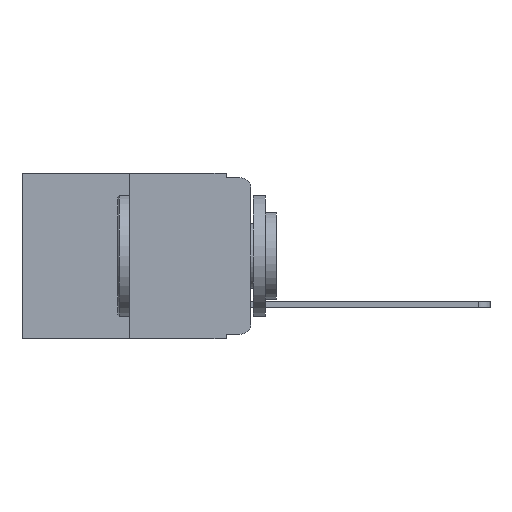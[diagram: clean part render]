
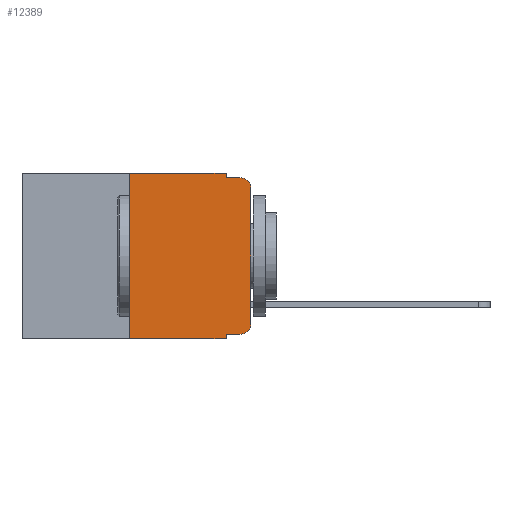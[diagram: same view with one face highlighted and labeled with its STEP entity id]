
A CAD part, left-side view. The second image highlights one B-rep face of the part: STEP entity #12389.
In plain terms, the highlighted planar face has unit normal (-1, 0, 0).
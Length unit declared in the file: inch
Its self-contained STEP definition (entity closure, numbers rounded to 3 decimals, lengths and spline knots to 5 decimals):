
#187 = ORIENTED_EDGE ( 'NONE', *, *, #15981, .F. ) ;
#561 = VECTOR ( 'NONE', #2764, 39.37008 ) ;
#1477 = DIRECTION ( 'NONE',  ( 0., 0., -1. ) ) ;
#1606 = ORIENTED_EDGE ( 'NONE', *, *, #15939, .F. ) ;
#1627 = LINE ( 'NONE', #7523, #6175 ) ;
#1663 = EDGE_CURVE ( 'NONE', #6163, #7898, #3650, .T. ) ;
#1715 = CARTESIAN_POINT ( 'NONE',  ( 0., 0.051, -0.01 ) ) ;
#2299 = CARTESIAN_POINT ( 'NONE',  ( 0., 0.051, -0.343 ) ) ;
#2764 = DIRECTION ( 'NONE',  ( 0., 0., -1. ) ) ;
#3650 = LINE ( 'NONE', #5828, #14278 ) ;
#4396 = ORIENTED_EDGE ( 'NONE', *, *, #6915, .F. ) ;
#5014 = VECTOR ( 'NONE', #7678, 39.37008 ) ;
#5183 = CARTESIAN_POINT ( 'NONE',  ( 0., 0., -0.313 ) ) ;
#5252 = EDGE_CURVE ( 'NONE', #21547, #19564, #20671, .T. ) ;
#5579 = ORIENTED_EDGE ( 'NONE', *, *, #14327, .T. ) ;
#5751 = DIRECTION ( 'NONE',  ( 0., -1., 0. ) ) ;
#5796 = CARTESIAN_POINT ( 'NONE',  ( 0., 0.25, 0. ) ) ;
#5828 = CARTESIAN_POINT ( 'NONE',  ( 0., 0.473, 0. ) ) ;
#5859 = LINE ( 'NONE', #10285, #561 ) ;
#5988 = LINE ( 'NONE', #23269, #15465 ) ;
#6163 = VERTEX_POINT ( 'NONE', #21907 ) ;
#6175 = VECTOR ( 'NONE', #9389, 39.37008 ) ;
#6274 = DIRECTION ( 'NONE',  ( 0., -1., 0. ) ) ;
#6359 = CARTESIAN_POINT ( 'NONE',  ( 0., 0., 0. ) ) ;
#6886 = CARTESIAN_POINT ( 'NONE',  ( 0., 0.051, -0.333 ) ) ;
#6915 = EDGE_CURVE ( 'NONE', #8893, #14971, #8928, .T. ) ;
#7220 = CARTESIAN_POINT ( 'NONE',  ( 0., 0.473, 0. ) ) ;
#7337 = CARTESIAN_POINT ( 'NONE',  ( 0., 0.25, -0.343 ) ) ;
#7523 = CARTESIAN_POINT ( 'NONE',  ( 0., 0.051, 0. ) ) ;
#7678 = DIRECTION ( 'NONE',  ( 0., 0., 1. ) ) ;
#7898 = VERTEX_POINT ( 'NONE', #15655 ) ;
#7917 = LINE ( 'NONE', #14983, #12435 ) ;
#8893 = VERTEX_POINT ( 'NONE', #1715 ) ;
#8928 = LINE ( 'NONE', #17516, #18314 ) ;
#9149 = DIRECTION ( 'NONE',  ( -1., 0., 0. ) ) ;
#9245 = DIRECTION ( 'NONE',  ( -1., 0., 0. ) ) ;
#9276 = VERTEX_POINT ( 'NONE', #18692 ) ;
#9389 = DIRECTION ( 'NONE',  ( 0., 0., -1. ) ) ;
#10231 = DIRECTION ( 'NONE',  ( 0., 0., 1. ) ) ;
#10285 = CARTESIAN_POINT ( 'NONE',  ( 0., 0.051, 0. ) ) ;
#10387 = CARTESIAN_POINT ( 'NONE',  ( 0., 0.02, -0.01 ) ) ;
#11276 = CIRCLE ( 'NONE', #22188, 0.02 ) ;
#11809 = ORIENTED_EDGE ( 'NONE', *, *, #15901, .T. ) ;
#12212 = CARTESIAN_POINT ( 'NONE',  ( 0., 0., -0.03 ) ) ;
#12389 = ADVANCED_FACE ( 'NONE', ( #17385 ), #23359, .F. ) ;
#12416 = ORIENTED_EDGE ( 'NONE', *, *, #15840, .T. ) ;
#12423 = EDGE_CURVE ( 'NONE', #19564, #14971, #11276, .T. ) ;
#12435 = VECTOR ( 'NONE', #16842, 39.37008 ) ;
#12580 = VERTEX_POINT ( 'NONE', #2299 ) ;
#12964 = DIRECTION ( 'NONE',  ( 1., 0., 0. ) ) ;
#14278 = VECTOR ( 'NONE', #5751, 39.37008 ) ;
#14327 = EDGE_CURVE ( 'NONE', #20483, #12580, #5988, .T. ) ;
#14447 = ORIENTED_EDGE ( 'NONE', *, *, #16163, .F. ) ;
#14739 = DIRECTION ( 'NONE',  ( 0., -1., 0. ) ) ;
#14971 = VERTEX_POINT ( 'NONE', #10387 ) ;
#14983 = CARTESIAN_POINT ( 'NONE',  ( 0., 0.051, -0.333 ) ) ;
#15042 = LINE ( 'NONE', #5796, #5014 ) ;
#15465 = VECTOR ( 'NONE', #14739, 39.37008 ) ;
#15655 = CARTESIAN_POINT ( 'NONE',  ( 0., 0.051, 0. ) ) ;
#15840 = EDGE_CURVE ( 'NONE', #9276, #21547, #22314, .T. ) ;
#15901 = EDGE_CURVE ( 'NONE', #19919, #9276, #7917, .T. ) ;
#15939 = EDGE_CURVE ( 'NONE', #19919, #12580, #1627, .T. ) ;
#15981 = EDGE_CURVE ( 'NONE', #20483, #6163, #15042, .T. ) ;
#16154 = VECTOR ( 'NONE', #10231, 39.37008 ) ;
#16163 = EDGE_CURVE ( 'NONE', #7898, #8893, #5859, .T. ) ;
#16787 = AXIS2_PLACEMENT_3D ( 'NONE', #20087, #9149, #21751 ) ;
#16842 = DIRECTION ( 'NONE',  ( 0., -1., 0. ) ) ;
#17385 = FACE_OUTER_BOUND ( 'NONE', #20539, .T. ) ;
#17516 = CARTESIAN_POINT ( 'NONE',  ( 0., 0.051, -0.01 ) ) ;
#18152 = ORIENTED_EDGE ( 'NONE', *, *, #5252, .T. ) ;
#18314 = VECTOR ( 'NONE', #6274, 39.37008 ) ;
#18692 = CARTESIAN_POINT ( 'NONE',  ( 0., 0.02, -0.333 ) ) ;
#19564 = VERTEX_POINT ( 'NONE', #12212 ) ;
#19919 = VERTEX_POINT ( 'NONE', #6886 ) ;
#20087 = CARTESIAN_POINT ( 'NONE',  ( 0., 0.02, -0.313 ) ) ;
#20175 = CARTESIAN_POINT ( 'NONE',  ( 0., 0.02, -0.03 ) ) ;
#20483 = VERTEX_POINT ( 'NONE', #7337 ) ;
#20539 = EDGE_LOOP ( 'NONE', ( #18152, #22555, #4396, #14447, #23543, #187, #5579, #1606, #11809, #12416 ) ) ;
#20671 = LINE ( 'NONE', #6359, #16154 ) ;
#21547 = VERTEX_POINT ( 'NONE', #5183 ) ;
#21751 = DIRECTION ( 'NONE',  ( 0., 0., -1. ) ) ;
#21853 = DIRECTION ( 'NONE',  ( 0., 0., -1. ) ) ;
#21907 = CARTESIAN_POINT ( 'NONE',  ( 0., 0.25, 0. ) ) ;
#22188 = AXIS2_PLACEMENT_3D ( 'NONE', #20175, #9245, #21853 ) ;
#22314 = CIRCLE ( 'NONE', #16787, 0.02 ) ;
#22555 = ORIENTED_EDGE ( 'NONE', *, *, #12423, .T. ) ;
#23269 = CARTESIAN_POINT ( 'NONE',  ( 0., 0.473, -0.343 ) ) ;
#23288 = AXIS2_PLACEMENT_3D ( 'NONE', #7220, #12964, #1477 ) ;
#23359 = PLANE ( 'NONE',  #23288 ) ;
#23543 = ORIENTED_EDGE ( 'NONE', *, *, #1663, .F. ) ;
